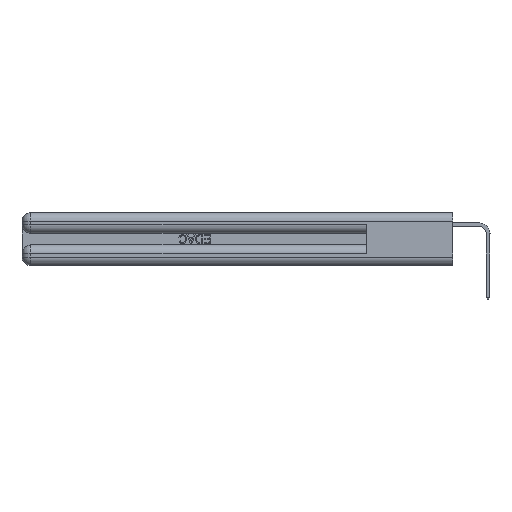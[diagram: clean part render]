
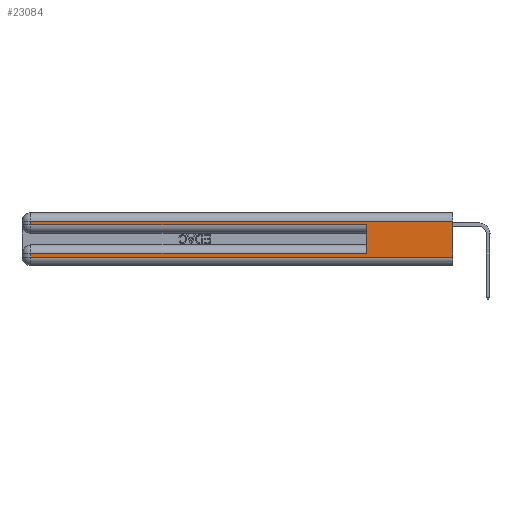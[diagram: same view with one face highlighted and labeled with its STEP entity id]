
A CAD part, left-side view. The second image highlights one B-rep face of the part: STEP entity #23084.
In plain terms, the highlighted planar face has unit normal (-1, 0, 0).
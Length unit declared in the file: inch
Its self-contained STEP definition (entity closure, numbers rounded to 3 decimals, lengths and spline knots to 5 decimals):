
#384 = CARTESIAN_POINT ( 'NONE',  ( 0., 2.94, 0.285 ) ) ;
#427 = CARTESIAN_POINT ( 'NONE',  ( 0., 0., 0.37 ) ) ;
#440 = EDGE_CURVE ( 'NONE', #40521, #25076, #11070, .T. ) ;
#452 = CARTESIAN_POINT ( 'NONE',  ( 0., 0.6, 0.145 ) ) ;
#458 = CARTESIAN_POINT ( 'NONE',  ( 0., 2.94, 0.31 ) ) ;
#928 = CARTESIAN_POINT ( 'NONE',  ( 0., 0., 0.37 ) ) ;
#1830 = DIRECTION ( 'NONE',  ( 0., 1., 0. ) ) ;
#2009 = VECTOR ( 'NONE', #38353, 39.37008 ) ;
#4542 = DIRECTION ( 'NONE',  ( 0., 0., -1. ) ) ;
#5113 = ORIENTED_EDGE ( 'NONE', *, *, #39690, .T. ) ;
#5142 = ORIENTED_EDGE ( 'NONE', *, *, #40674, .F. ) ;
#5251 = VECTOR ( 'NONE', #33414, 39.37008 ) ;
#5255 = CARTESIAN_POINT ( 'NONE',  ( 0., 0., 0.085 ) ) ;
#5650 = DIRECTION ( 'NONE',  ( 0., -1., 0. ) ) ;
#5672 = VECTOR ( 'NONE', #5650, 39.37008 ) ;
#7643 = VERTEX_POINT ( 'NONE', #20643 ) ;
#7777 = DIRECTION ( 'NONE',  ( 1., 0., 0. ) ) ;
#8485 = VERTEX_POINT ( 'NONE', #384 ) ;
#11070 = LINE ( 'NONE', #31456, #2009 ) ;
#11891 = ORIENTED_EDGE ( 'NONE', *, *, #440, .T. ) ;
#12881 = CARTESIAN_POINT ( 'NONE',  ( 0., 0.6, 0.285 ) ) ;
#13478 = EDGE_CURVE ( 'NONE', #24320, #40521, #20582, .T. ) ;
#14264 = LINE ( 'NONE', #32618, #15327 ) ;
#15125 = LINE ( 'NONE', #452, #23150 ) ;
#15327 = VECTOR ( 'NONE', #1830, 39.37008 ) ;
#16444 = CARTESIAN_POINT ( 'NONE',  ( 0., 0., 0.31 ) ) ;
#17429 = DIRECTION ( 'NONE',  ( 0., 0., -1. ) ) ;
#18193 = VERTEX_POINT ( 'NONE', #458 ) ;
#20582 = LINE ( 'NONE', #5255, #28612 ) ;
#20643 = CARTESIAN_POINT ( 'NONE',  ( 0., 0., 0.06 ) ) ;
#21178 = AXIS2_PLACEMENT_3D ( 'NONE', #928, #7777, #31713 ) ;
#22982 = CARTESIAN_POINT ( 'NONE',  ( 0., 2.94, 0.06 ) ) ;
#23084 = ADVANCED_FACE ( 'NONE', ( #37291 ), #31563, .F. ) ;
#23150 = VECTOR ( 'NONE', #34560, 39.37008 ) ;
#23379 = LINE ( 'NONE', #42065, #31431 ) ;
#23567 = ORIENTED_EDGE ( 'NONE', *, *, #40326, .T. ) ;
#24015 = VERTEX_POINT ( 'NONE', #12881 ) ;
#24320 = VERTEX_POINT ( 'NONE', #41773 ) ;
#25076 = VERTEX_POINT ( 'NONE', #22982 ) ;
#25972 = VECTOR ( 'NONE', #17429, 39.37008 ) ;
#26142 = CARTESIAN_POINT ( 'NONE',  ( 0., 0., 0.285 ) ) ;
#28057 = ORIENTED_EDGE ( 'NONE', *, *, #32158, .T. ) ;
#28612 = VECTOR ( 'NONE', #36089, 39.37008 ) ;
#29330 = ORIENTED_EDGE ( 'NONE', *, *, #39227, .T. ) ;
#29947 = CARTESIAN_POINT ( 'NONE',  ( 0., 0., 0.06 ) ) ;
#30403 = ORIENTED_EDGE ( 'NONE', *, *, #36413, .F. ) ;
#30600 = VERTEX_POINT ( 'NONE', #16444 ) ;
#31431 = VECTOR ( 'NONE', #4542, 39.37008 ) ;
#31456 = CARTESIAN_POINT ( 'NONE',  ( 0., 2.94, 0.37 ) ) ;
#31563 = PLANE ( 'NONE',  #21178 ) ;
#31713 = DIRECTION ( 'NONE',  ( 0., 0., -1. ) ) ;
#31912 = LINE ( 'NONE', #26142, #5672 ) ;
#32158 = EDGE_CURVE ( 'NONE', #30600, #18193, #14264, .T. ) ;
#32618 = CARTESIAN_POINT ( 'NONE',  ( 0., 0., 0.31 ) ) ;
#33414 = DIRECTION ( 'NONE',  ( 0., -1., 0. ) ) ;
#34560 = DIRECTION ( 'NONE',  ( 0., 0., 1. ) ) ;
#34736 = LINE ( 'NONE', #29947, #5251 ) ;
#36089 = DIRECTION ( 'NONE',  ( 0., 1., 0. ) ) ;
#36090 = EDGE_LOOP ( 'NONE', ( #5142, #28057, #5113, #23567, #30403, #41730, #11891, #29330 ) ) ;
#36413 = EDGE_CURVE ( 'NONE', #24320, #24015, #15125, .T. ) ;
#37217 = CARTESIAN_POINT ( 'NONE',  ( 0., 2.94, 0.085 ) ) ;
#37291 = FACE_OUTER_BOUND ( 'NONE', #36090, .T. ) ;
#38353 = DIRECTION ( 'NONE',  ( 0., 0., -1. ) ) ;
#39227 = EDGE_CURVE ( 'NONE', #25076, #7643, #34736, .T. ) ;
#39690 = EDGE_CURVE ( 'NONE', #18193, #8485, #23379, .T. ) ;
#40326 = EDGE_CURVE ( 'NONE', #8485, #24015, #31912, .T. ) ;
#40521 = VERTEX_POINT ( 'NONE', #37217 ) ;
#40674 = EDGE_CURVE ( 'NONE', #30600, #7643, #44173, .T. ) ;
#41730 = ORIENTED_EDGE ( 'NONE', *, *, #13478, .T. ) ;
#41773 = CARTESIAN_POINT ( 'NONE',  ( 0., 0.6, 0.085 ) ) ;
#42065 = CARTESIAN_POINT ( 'NONE',  ( 0., 2.94, 0.37 ) ) ;
#44173 = LINE ( 'NONE', #427, #25972 ) ;
